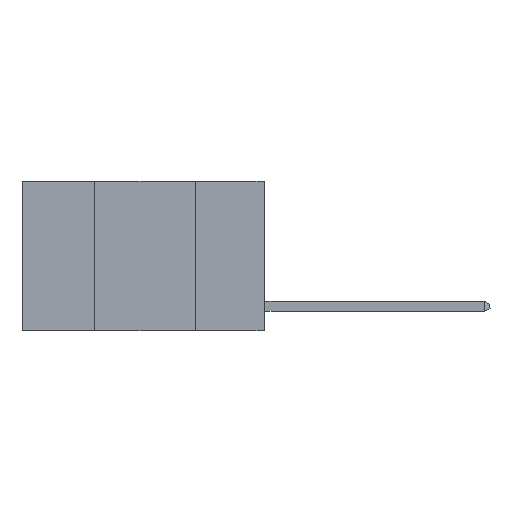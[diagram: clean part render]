
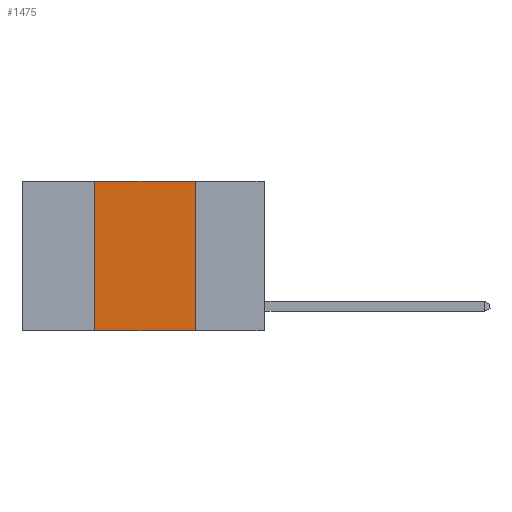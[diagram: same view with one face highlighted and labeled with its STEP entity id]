
A CAD part, left-side view. The second image highlights one B-rep face of the part: STEP entity #1475.
In plain terms, the highlighted planar face has unit normal (-1, 0, 0).
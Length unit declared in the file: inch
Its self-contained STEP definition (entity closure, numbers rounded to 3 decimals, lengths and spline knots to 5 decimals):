
#213 = ORIENTED_EDGE ( 'NONE', *, *, #1005, .T. ) ;
#783 = CARTESIAN_POINT ( 'NONE',  ( 0., 0.42, 0. ) ) ;
#883 = ORIENTED_EDGE ( 'NONE', *, *, #7602, .F. ) ;
#901 = CARTESIAN_POINT ( 'NONE',  ( 0., 0.6, -0.37 ) ) ;
#977 = DIRECTION ( 'NONE',  ( 0., 0., -1. ) ) ;
#1005 = EDGE_CURVE ( 'NONE', #3355, #2882, #4645, .T. ) ;
#1201 = CARTESIAN_POINT ( 'NONE',  ( 0., 0.17, -0.37 ) ) ;
#1316 = VECTOR ( 'NONE', #5712, 39.37008 ) ;
#1475 = ADVANCED_FACE ( 'NONE', ( #6927 ), #8939, .F. ) ;
#1631 = CARTESIAN_POINT ( 'NONE',  ( 0., 0.42, -0.37 ) ) ;
#1936 = CARTESIAN_POINT ( 'NONE',  ( 0., 0.17, 0. ) ) ;
#2649 = AXIS2_PLACEMENT_3D ( 'NONE', #4580, #7453, #977 ) ;
#2695 = EDGE_CURVE ( 'NONE', #3355, #8005, #3584, .T. ) ;
#2831 = CARTESIAN_POINT ( 'NONE',  ( 0., 0.42, 0. ) ) ;
#2882 = VERTEX_POINT ( 'NONE', #1201 ) ;
#3355 = VERTEX_POINT ( 'NONE', #1631 ) ;
#3388 = VECTOR ( 'NONE', #7467, 39.37008 ) ;
#3504 = DIRECTION ( 'NONE',  ( 0., -1., 0. ) ) ;
#3550 = ORIENTED_EDGE ( 'NONE', *, *, #8248, .F. ) ;
#3584 = LINE ( 'NONE', #2831, #1316 ) ;
#4472 = VECTOR ( 'NONE', #8432, 39.37008 ) ;
#4580 = CARTESIAN_POINT ( 'NONE',  ( 0., 0.6, 0. ) ) ;
#4645 = LINE ( 'NONE', #901, #3388 ) ;
#5712 = DIRECTION ( 'NONE',  ( 0., 0., 1. ) ) ;
#5816 = VECTOR ( 'NONE', #3504, 39.37008 ) ;
#5955 = EDGE_LOOP ( 'NONE', ( #3550, #883, #6511, #213 ) ) ;
#6162 = VERTEX_POINT ( 'NONE', #7756 ) ;
#6511 = ORIENTED_EDGE ( 'NONE', *, *, #2695, .F. ) ;
#6927 = FACE_OUTER_BOUND ( 'NONE', #5955, .T. ) ;
#7005 = LINE ( 'NONE', #1936, #4472 ) ;
#7087 = CARTESIAN_POINT ( 'NONE',  ( 0., 0.6, 0. ) ) ;
#7453 = DIRECTION ( 'NONE',  ( 1., 0., 0. ) ) ;
#7467 = DIRECTION ( 'NONE',  ( 0., -1., 0. ) ) ;
#7602 = EDGE_CURVE ( 'NONE', #8005, #6162, #9072, .T. ) ;
#7756 = CARTESIAN_POINT ( 'NONE',  ( 0., 0.17, 0. ) ) ;
#8005 = VERTEX_POINT ( 'NONE', #783 ) ;
#8248 = EDGE_CURVE ( 'NONE', #6162, #2882, #7005, .T. ) ;
#8432 = DIRECTION ( 'NONE',  ( 0., 0., -1. ) ) ;
#8939 = PLANE ( 'NONE',  #2649 ) ;
#9072 = LINE ( 'NONE', #7087, #5816 ) ;
